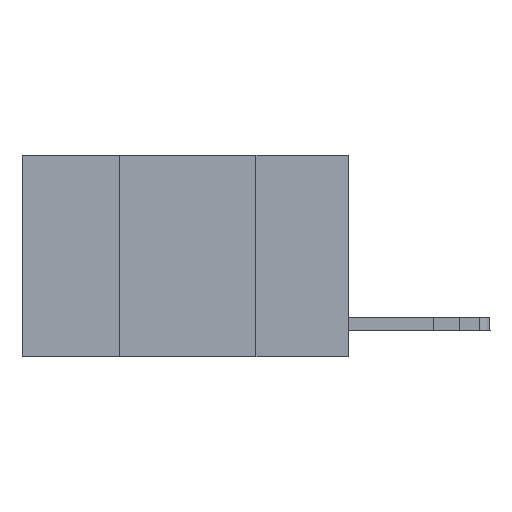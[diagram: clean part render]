
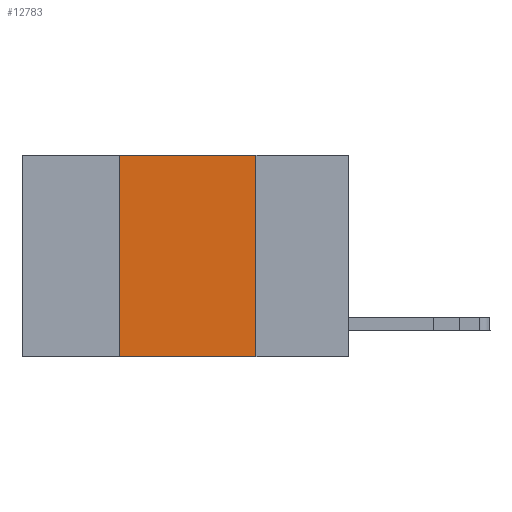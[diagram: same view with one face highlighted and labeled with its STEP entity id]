
A CAD part, left-side view. The second image highlights one B-rep face of the part: STEP entity #12783.
In plain terms, the highlighted planar face has unit normal (-1, 0, 0).
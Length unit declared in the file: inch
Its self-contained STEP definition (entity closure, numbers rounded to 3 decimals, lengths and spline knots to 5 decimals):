
#427 = CARTESIAN_POINT ( 'NONE',  ( 0., 0.6, -0.37 ) ) ;
#955 = ORIENTED_EDGE ( 'NONE', *, *, #22507, .F. ) ;
#1417 = PLANE ( 'NONE',  #5223 ) ;
#1743 = CARTESIAN_POINT ( 'NONE',  ( 0., 0.17, -0.37 ) ) ;
#2511 = DIRECTION ( 'NONE',  ( 0., -1., 0. ) ) ;
#3647 = ORIENTED_EDGE ( 'NONE', *, *, #6820, .F. ) ;
#3698 = LINE ( 'NONE', #17786, #9503 ) ;
#5223 = AXIS2_PLACEMENT_3D ( 'NONE', #14893, #19126, #18895 ) ;
#5237 = VERTEX_POINT ( 'NONE', #1743 ) ;
#5722 = VECTOR ( 'NONE', #18035, 39.37008 ) ;
#6222 = VERTEX_POINT ( 'NONE', #16128 ) ;
#6381 = CARTESIAN_POINT ( 'NONE',  ( 0., 0.42, 0. ) ) ;
#6640 = VECTOR ( 'NONE', #2511, 39.37008 ) ;
#6820 = EDGE_CURVE ( 'NONE', #6222, #15078, #10022, .T. ) ;
#7782 = ORIENTED_EDGE ( 'NONE', *, *, #19443, .T. ) ;
#9350 = CARTESIAN_POINT ( 'NONE',  ( 0., 0.42, -0.37 ) ) ;
#9503 = VECTOR ( 'NONE', #23101, 39.37008 ) ;
#10008 = EDGE_CURVE ( 'NONE', #15078, #5237, #3698, .T. ) ;
#10022 = LINE ( 'NONE', #23835, #6640 ) ;
#11232 = CARTESIAN_POINT ( 'NONE',  ( 0., 0.17, 0. ) ) ;
#12395 = EDGE_LOOP ( 'NONE', ( #14330, #3647, #955, #7782 ) ) ;
#12783 = ADVANCED_FACE ( 'NONE', ( #15246 ), #1417, .F. ) ;
#14093 = DIRECTION ( 'NONE',  ( 0., 0., 1. ) ) ;
#14312 = VERTEX_POINT ( 'NONE', #9350 ) ;
#14330 = ORIENTED_EDGE ( 'NONE', *, *, #10008, .F. ) ;
#14893 = CARTESIAN_POINT ( 'NONE',  ( 0., 0.6, 0. ) ) ;
#15078 = VERTEX_POINT ( 'NONE', #11232 ) ;
#15246 = FACE_OUTER_BOUND ( 'NONE', #12395, .T. ) ;
#16128 = CARTESIAN_POINT ( 'NONE',  ( 0., 0.42, 0. ) ) ;
#17786 = CARTESIAN_POINT ( 'NONE',  ( 0., 0.17, 0. ) ) ;
#18035 = DIRECTION ( 'NONE',  ( 0., -1., 0. ) ) ;
#18895 = DIRECTION ( 'NONE',  ( 0., 0., -1. ) ) ;
#19126 = DIRECTION ( 'NONE',  ( 1., 0., 0. ) ) ;
#19443 = EDGE_CURVE ( 'NONE', #14312, #5237, #21457, .T. ) ;
#21457 = LINE ( 'NONE', #427, #5722 ) ;
#22507 = EDGE_CURVE ( 'NONE', #14312, #6222, #23698, .T. ) ;
#23101 = DIRECTION ( 'NONE',  ( 0., 0., -1. ) ) ;
#23698 = LINE ( 'NONE', #6381, #24726 ) ;
#23835 = CARTESIAN_POINT ( 'NONE',  ( 0., 0.6, 0. ) ) ;
#24726 = VECTOR ( 'NONE', #14093, 39.37008 ) ;
